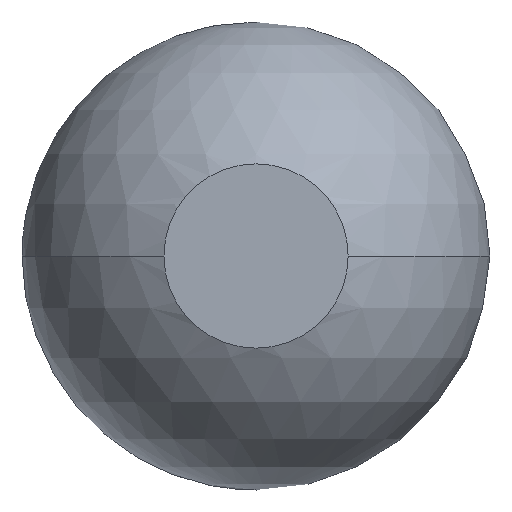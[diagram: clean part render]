
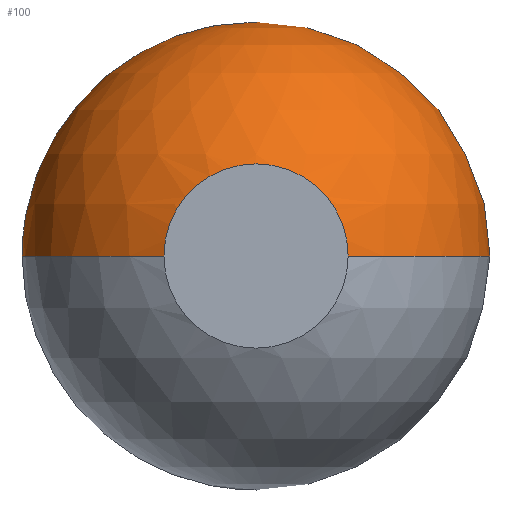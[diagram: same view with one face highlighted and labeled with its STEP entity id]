
A CAD part, front view. The second image highlights one B-rep face of the part: STEP entity #100.
In plain terms, the highlighted spherical face has radius 3.81 mm.
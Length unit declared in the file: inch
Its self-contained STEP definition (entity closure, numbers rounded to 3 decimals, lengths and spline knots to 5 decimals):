
#11 = DIRECTION ( 'NONE',  ( -1., 0., 0. ) ) ;
#18 = AXIS2_PLACEMENT_3D ( 'NONE', #76, #26, #75 ) ;
#23 = DIRECTION ( 'NONE',  ( 0., 0., -1. ) ) ;
#26 = DIRECTION ( 'NONE',  ( 0., 0., -1. ) ) ;
#28 = DIRECTION ( 'NONE',  ( 1., 0., 0. ) ) ;
#31 = CARTESIAN_POINT ( 'NONE',  ( 0., 0.88789, 0. ) ) ;
#49 = VERTEX_POINT ( 'NONE', #163 ) ;
#53 = AXIS2_PLACEMENT_3D ( 'NONE', #165, #23, #11 ) ;
#58 = SPHERICAL_SURFACE ( 'NONE', #53, 0.15 ) ;
#75 = DIRECTION ( 'NONE',  ( -1., 0., 0. ) ) ;
#76 = CARTESIAN_POINT ( 'NONE',  ( 0., 0.88789, 0. ) ) ;
#81 = DIRECTION ( 'NONE',  ( 0., 0., 1. ) ) ;
#86 = CARTESIAN_POINT ( 'NONE',  ( 0.05906, 0.75, 0. ) ) ;
#87 = CARTESIAN_POINT ( 'NONE',  ( 0., 1.03789, 0. ) ) ;
#92 = AXIS2_PLACEMENT_3D ( 'NONE', #104, #110, #120 ) ;
#99 = FACE_OUTER_BOUND ( 'NONE', #126, .T. ) ;
#100 = ADVANCED_FACE ( 'NONE', ( #99 ), #58, .T. ) ;
#102 = EDGE_CURVE ( 'NONE', #131, #49, #113, .T. ) ;
#104 = CARTESIAN_POINT ( 'NONE',  ( 0., 0.75, 0. ) ) ;
#105 = ORIENTED_EDGE ( 'NONE', *, *, #146, .T. ) ;
#110 = DIRECTION ( 'NONE',  ( 0., -1., 0. ) ) ;
#113 = CIRCLE ( 'NONE', #92, 0.05906 ) ;
#120 = DIRECTION ( 'NONE',  ( 1., 0., 0. ) ) ;
#124 = ORIENTED_EDGE ( 'NONE', *, *, #170, .F. ) ;
#126 = EDGE_LOOP ( 'NONE', ( #124, #105, #166 ) ) ;
#130 = VERTEX_POINT ( 'NONE', #87 ) ;
#131 = VERTEX_POINT ( 'NONE', #86 ) ;
#143 = AXIS2_PLACEMENT_3D ( 'NONE', #31, #81, #28 ) ;
#145 = CIRCLE ( 'NONE', #143, 0.15 ) ;
#146 = EDGE_CURVE ( 'NONE', #130, #49, #145, .T. ) ;
#161 = CIRCLE ( 'NONE', #18, 0.15 ) ;
#163 = CARTESIAN_POINT ( 'NONE',  ( -0.05906, 0.75, 0. ) ) ;
#165 = CARTESIAN_POINT ( 'NONE',  ( 0., 0.88789, 0. ) ) ;
#166 = ORIENTED_EDGE ( 'NONE', *, *, #102, .F. ) ;
#170 = EDGE_CURVE ( 'NONE', #130, #131, #161, .T. ) ;
